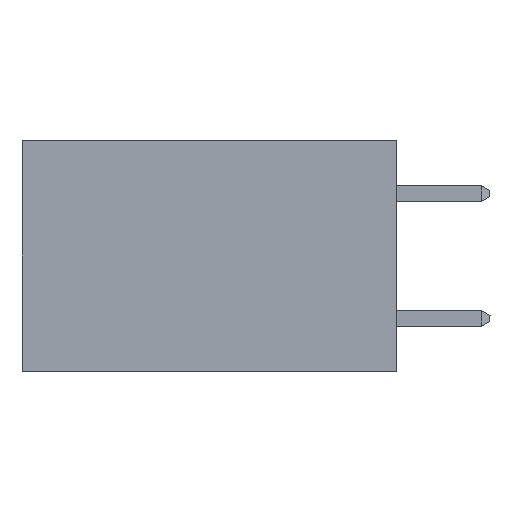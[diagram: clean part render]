
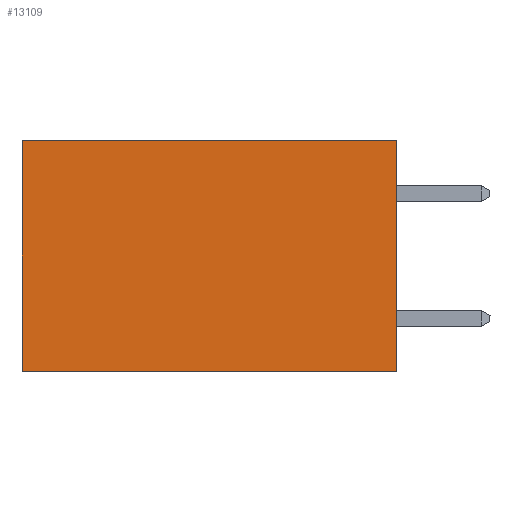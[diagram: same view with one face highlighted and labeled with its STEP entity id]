
A CAD part, left-side view. The second image highlights one B-rep face of the part: STEP entity #13109.
In plain terms, the highlighted planar face has unit normal (-1, 0, 0).
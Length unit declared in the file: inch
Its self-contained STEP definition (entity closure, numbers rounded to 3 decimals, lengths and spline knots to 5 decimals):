
#925 = CARTESIAN_POINT ( 'NONE',  ( 0.298, 0., 0. ) ) ;
#2217 = EDGE_CURVE ( 'NONE', #7790, #17163, #15431, .T. ) ;
#2300 = DIRECTION ( 'NONE',  ( 0., 1., 0. ) ) ;
#2503 = CARTESIAN_POINT ( 'NONE',  ( 0.298, 0., -0.37 ) ) ;
#2908 = EDGE_CURVE ( 'NONE', #17977, #20984, #22650, .T. ) ;
#2968 = AXIS2_PLACEMENT_3D ( 'NONE', #16539, #5296, #11061 ) ;
#3835 = ORIENTED_EDGE ( 'NONE', *, *, #19066, .F. ) ;
#4792 = CARTESIAN_POINT ( 'NONE',  ( 0.298, 0.6, 0. ) ) ;
#5296 = DIRECTION ( 'NONE',  ( 1., 0., 0. ) ) ;
#6067 = ORIENTED_EDGE ( 'NONE', *, *, #2217, .F. ) ;
#6643 = CARTESIAN_POINT ( 'NONE',  ( 0.298, 0., -0.37 ) ) ;
#7790 = VERTEX_POINT ( 'NONE', #15139 ) ;
#8540 = DIRECTION ( 'NONE',  ( 0., 0., -1. ) ) ;
#9454 = EDGE_CURVE ( 'NONE', #7790, #17977, #19602, .T. ) ;
#11061 = DIRECTION ( 'NONE',  ( 0., 0., -1. ) ) ;
#11818 = VECTOR ( 'NONE', #2300, 39.37008 ) ;
#12244 = ORIENTED_EDGE ( 'NONE', *, *, #2908, .T. ) ;
#12726 = EDGE_LOOP ( 'NONE', ( #12244, #3835, #6067, #17955 ) ) ;
#12829 = PLANE ( 'NONE',  #2968 ) ;
#13109 = ADVANCED_FACE ( 'NONE', ( #19164 ), #12829, .F. ) ;
#15139 = CARTESIAN_POINT ( 'NONE',  ( 0.298, 0., 0. ) ) ;
#15380 = DIRECTION ( 'NONE',  ( 0., 1., 0. ) ) ;
#15431 = LINE ( 'NONE', #925, #20624 ) ;
#15793 = VECTOR ( 'NONE', #15380, 39.37008 ) ;
#16539 = CARTESIAN_POINT ( 'NONE',  ( 0.298, 0., 0. ) ) ;
#16563 = VECTOR ( 'NONE', #8540, 39.37008 ) ;
#17163 = VERTEX_POINT ( 'NONE', #6643 ) ;
#17955 = ORIENTED_EDGE ( 'NONE', *, *, #9454, .T. ) ;
#17977 = VERTEX_POINT ( 'NONE', #4792 ) ;
#19066 = EDGE_CURVE ( 'NONE', #17163, #20984, #21300, .T. ) ;
#19133 = DIRECTION ( 'NONE',  ( 0., 0., -1. ) ) ;
#19164 = FACE_OUTER_BOUND ( 'NONE', #12726, .T. ) ;
#19352 = CARTESIAN_POINT ( 'NONE',  ( 0.298, 0.6, -0.37 ) ) ;
#19602 = LINE ( 'NONE', #20500, #11818 ) ;
#20500 = CARTESIAN_POINT ( 'NONE',  ( 0.298, 0., 0. ) ) ;
#20624 = VECTOR ( 'NONE', #19133, 39.37008 ) ;
#20984 = VERTEX_POINT ( 'NONE', #19352 ) ;
#21300 = LINE ( 'NONE', #2503, #15793 ) ;
#22650 = LINE ( 'NONE', #23403, #16563 ) ;
#23403 = CARTESIAN_POINT ( 'NONE',  ( 0.298, 0.6, 0. ) ) ;
